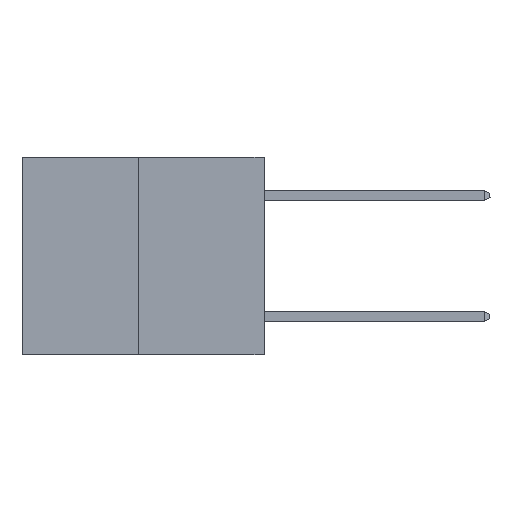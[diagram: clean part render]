
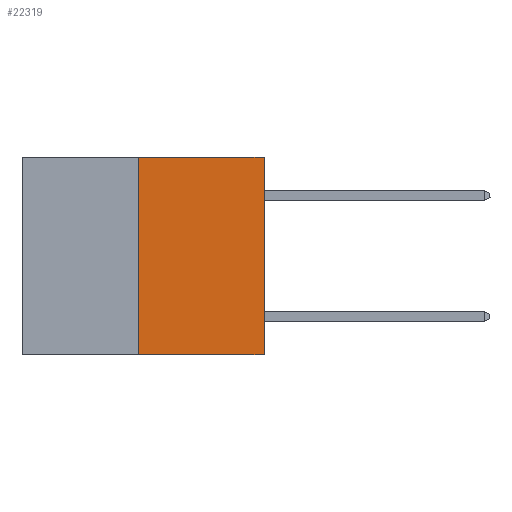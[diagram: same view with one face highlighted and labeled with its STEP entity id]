
A CAD part, left-side view. The second image highlights one B-rep face of the part: STEP entity #22319.
In plain terms, the highlighted planar face has unit normal (-1, 0, 0).
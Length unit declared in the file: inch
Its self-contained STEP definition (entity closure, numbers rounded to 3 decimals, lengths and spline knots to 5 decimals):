
#993 = VECTOR ( 'NONE', #13254, 39.37008 ) ;
#1796 = DIRECTION ( 'NONE',  ( 0., 0., -1. ) ) ;
#3011 = ORIENTED_EDGE ( 'NONE', *, *, #24943, .F. ) ;
#4467 = LINE ( 'NONE', #14863, #22778 ) ;
#5393 = CARTESIAN_POINT ( 'NONE',  ( 0., 0., 0. ) ) ;
#7333 = DIRECTION ( 'NONE',  ( 1., 0., 0. ) ) ;
#8992 = DIRECTION ( 'NONE',  ( 0., 0., 1. ) ) ;
#9012 = ORIENTED_EDGE ( 'NONE', *, *, #17988, .T. ) ;
#9787 = LINE ( 'NONE', #15012, #24989 ) ;
#12227 = ORIENTED_EDGE ( 'NONE', *, *, #18919, .T. ) ;
#13254 = DIRECTION ( 'NONE',  ( 0., 0., 1. ) ) ;
#13612 = PLANE ( 'NONE',  #24780 ) ;
#13804 = VERTEX_POINT ( 'NONE', #19421 ) ;
#14863 = CARTESIAN_POINT ( 'NONE',  ( 0., 0.6, 0. ) ) ;
#14958 = EDGE_LOOP ( 'NONE', ( #3011, #9012, #12227, #23028 ) ) ;
#15012 = CARTESIAN_POINT ( 'NONE',  ( 0., 0.6, -0.49 ) ) ;
#15669 = CARTESIAN_POINT ( 'NONE',  ( 0., 0.312, -0.49 ) ) ;
#16206 = EDGE_CURVE ( 'NONE', #13804, #25396, #4467, .T. ) ;
#17456 = LINE ( 'NONE', #19126, #21537 ) ;
#17988 = EDGE_CURVE ( 'NONE', #24556, #21069, #9787, .T. ) ;
#18140 = FACE_OUTER_BOUND ( 'NONE', #14958, .T. ) ;
#18919 = EDGE_CURVE ( 'NONE', #21069, #25396, #17456, .T. ) ;
#19126 = CARTESIAN_POINT ( 'NONE',  ( 0., 0., 0. ) ) ;
#19421 = CARTESIAN_POINT ( 'NONE',  ( 0., 0.312, 0. ) ) ;
#21069 = VERTEX_POINT ( 'NONE', #22589 ) ;
#21537 = VECTOR ( 'NONE', #8992, 39.37008 ) ;
#22319 = ADVANCED_FACE ( 'NONE', ( #18140 ), #13612, .F. ) ;
#22589 = CARTESIAN_POINT ( 'NONE',  ( 0., 0., -0.49 ) ) ;
#22778 = VECTOR ( 'NONE', #24798, 39.37008 ) ;
#23028 = ORIENTED_EDGE ( 'NONE', *, *, #16206, .F. ) ;
#23123 = CARTESIAN_POINT ( 'NONE',  ( 0., 0.312, -0.49 ) ) ;
#23347 = LINE ( 'NONE', #23123, #993 ) ;
#24556 = VERTEX_POINT ( 'NONE', #15669 ) ;
#24780 = AXIS2_PLACEMENT_3D ( 'NONE', #25271, #7333, #1796 ) ;
#24798 = DIRECTION ( 'NONE',  ( 0., -1., 0. ) ) ;
#24934 = DIRECTION ( 'NONE',  ( 0., -1., 0. ) ) ;
#24943 = EDGE_CURVE ( 'NONE', #24556, #13804, #23347, .T. ) ;
#24989 = VECTOR ( 'NONE', #24934, 39.37008 ) ;
#25271 = CARTESIAN_POINT ( 'NONE',  ( 0., 0.6, 0. ) ) ;
#25396 = VERTEX_POINT ( 'NONE', #5393 ) ;
